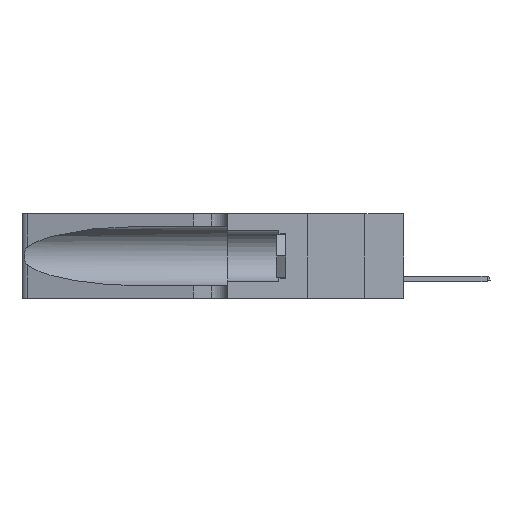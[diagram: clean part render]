
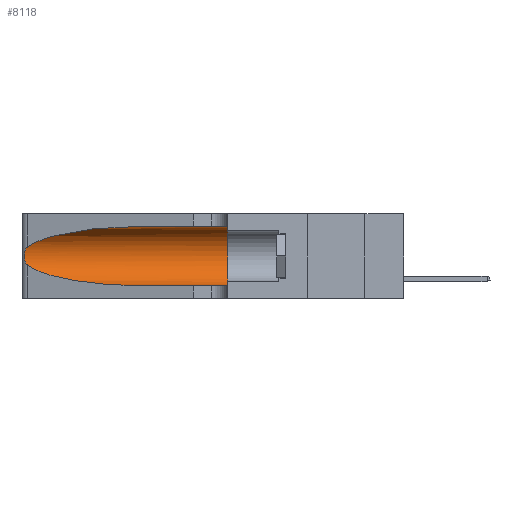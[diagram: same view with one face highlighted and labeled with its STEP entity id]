
A CAD part, left-side view. The second image highlights one B-rep face of the part: STEP entity #8118.
In plain terms, the highlighted cylindrical face has radius 3.308 mm (diameter 6.617 mm), a partial arc.
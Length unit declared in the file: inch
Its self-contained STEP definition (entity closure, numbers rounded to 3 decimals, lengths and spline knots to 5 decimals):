
#2579 = DIRECTION ( 'NONE',  ( 0., 1., 0. ) ) ;
#3588 = CARTESIAN_POINT ( 'NONE',  ( 0.1305, 0.72297, 0.05475 ) ) ;
#4040 = CARTESIAN_POINT ( 'NONE',  ( 0.1305, 0.72297, 0.31525 ) ) ;
#5181 = VECTOR ( 'NONE', #47254, 39.37008 ) ;
#6050 = CARTESIAN_POINT ( 'NONE',  ( 0.1305, 0.72297, 0.05475 ) ) ;
#7114 = EDGE_CURVE ( 'NONE', #20195, #26849, #46131, .T. ) ;
#7661 = CARTESIAN_POINT ( 'NONE',  ( 0.25639, 1.23186, 0.15144 ) ) ;
#7807 = CARTESIAN_POINT ( 'NONE',  ( 0.25555, 1.22994, 0.2215 ) ) ;
#8118 = ADVANCED_FACE ( 'NONE', ( #21408 ), #11809, .F. ) ;
#10130 = DIRECTION ( 'NONE',  ( 0., -1., 0. ) ) ;
#10303 = DIRECTION ( 'NONE',  ( 0., 0., -1. ) ) ;
#10623 = LINE ( 'NONE', #37215, #5181 ) ;
#10801 = CARTESIAN_POINT ( 'NONE',  ( 0.1305, 1.61858, 0.185 ) ) ;
#11359 = AXIS2_PLACEMENT_3D ( 'NONE', #10801, #10130, #10303 ) ;
#11375 = CARTESIAN_POINT ( 'NONE',  ( 0.26018, 1.23835, 0.19895 ) ) ;
#11809 = CYLINDRICAL_SURFACE ( 'NONE', #11359, 0.13025 ) ;
#12866 = EDGE_CURVE ( 'NONE', #38710, #25687, #27312, .T. ) ;
#13555 = EDGE_CURVE ( 'NONE', #47282, #38710, #10623, .T. ) ;
#14441 = CARTESIAN_POINT ( 'NONE',  ( 0.1305, 0.35, 0.185 ) ) ;
#15513 = CARTESIAN_POINT ( 'NONE',  ( 0.25555, 1.22993, 0.14849 ) ) ;
#16202 = ORIENTED_EDGE ( 'NONE', *, *, #36908, .T. ) ;
#17821 = VERTEX_POINT ( 'NONE', #40874 ) ;
#18726 = CARTESIAN_POINT ( 'NONE',  ( 0.26075, 1.23896, 0.178 ) ) ;
#18804 = CARTESIAN_POINT ( 'NONE',  ( 0.25487, 1.22718, 0.14631 ) ) ;
#19096 = CARTESIAN_POINT ( 'NONE',  ( 0.25487, 1.22718, 0.14631 ) ) ;
#19458 = CARTESIAN_POINT ( 'NONE',  ( 0.1305, 0.72297, 0.31525 ) ) ;
#20195 = VERTEX_POINT ( 'NONE', #19096 ) ;
#20687 = EDGE_CURVE ( 'NONE', #26849, #25687, #41101, .T. ) ;
#20751 = ORIENTED_EDGE ( 'NONE', *, *, #41582, .T. ) ;
#21408 = FACE_OUTER_BOUND ( 'NONE', #22323, .T. ) ;
#21809 = ORIENTED_EDGE ( 'NONE', *, *, #7114, .T. ) ;
#21927 = DIRECTION ( 'NONE',  ( 0., -1., 0. ) ) ;
#22323 = EDGE_LOOP ( 'NONE', ( #16202, #20751, #21809, #41801, #33899, #41941 ) ) ;
#22725 = CARTESIAN_POINT ( 'NONE',  ( 0.26017, 1.23833, 0.17102 ) ) ;
#24519 = CARTESIAN_POINT ( 'NONE',  ( 0.25487, 1.22718, 0.22369 ) ) ;
#25687 = VERTEX_POINT ( 'NONE', #37217 ) ;
#26424 = CARTESIAN_POINT ( 'NONE',  ( 0.18966, 0.96281, 0.05475 ) ) ;
#26512 = CARTESIAN_POINT ( 'NONE',  ( 0.25854, 1.2359, 0.20912 ) ) ;
#26849 = VERTEX_POINT ( 'NONE', #6050 ) ;
#26874 = CARTESIAN_POINT ( 'NONE',  ( 0.2373, 1.15595, 0.28018 ) ) ;
#27312 = CIRCLE ( 'NONE', #49216, 0.13025 ) ;
#30634 = CARTESIAN_POINT ( 'NONE',  ( 0.25487, 1.22718, 0.22369 ) ) ;
#32084 =( BOUNDED_CURVE ( )  B_SPLINE_CURVE ( 3, ( #19458, #46316, #26874, #24519 ),
 .UNSPECIFIED., .F., .T. ) 
 B_SPLINE_CURVE_WITH_KNOTS ( ( 4, 4 ),
 ( 1.5708, 2.84003 ),
 .UNSPECIFIED. ) 
 CURVE ( )  GEOMETRIC_REPRESENTATION_ITEM ( )  RATIONAL_B_SPLINE_CURVE ( ( 1., 0.87, 0.87, 1. ) ) 
 REPRESENTATION_ITEM ( '' )  );
#32607 = CARTESIAN_POINT ( 'NONE',  ( 0.1305, 0.35, 0.31525 ) ) ;
#33233 = CARTESIAN_POINT ( 'NONE',  ( 0.1305, 1.61858, 0.05475 ) ) ;
#33868 = CARTESIAN_POINT ( 'NONE',  ( 0.25639, 1.23184, 0.21858 ) ) ;
#33899 = ORIENTED_EDGE ( 'NONE', *, *, #12866, .F. ) ;
#36908 = EDGE_CURVE ( 'NONE', #47282, #17821, #32084, .T. ) ;
#37215 = CARTESIAN_POINT ( 'NONE',  ( 0.1305, 1.61858, 0.31525 ) ) ;
#37217 = CARTESIAN_POINT ( 'NONE',  ( 0.1305, 0.35, 0.05475 ) ) ;
#38016 = CARTESIAN_POINT ( 'NONE',  ( 0.25856, 1.23593, 0.16098 ) ) ;
#38341 = CARTESIAN_POINT ( 'NONE',  ( 0.25787, 1.23484, 0.2124 ) ) ;
#38710 = VERTEX_POINT ( 'NONE', #32607 ) ;
#40874 = CARTESIAN_POINT ( 'NONE',  ( 0.25487, 1.22718, 0.22369 ) ) ;
#41099 = DIRECTION ( 'NONE',  ( 0., 0., 1. ) ) ;
#41101 = LINE ( 'NONE', #33233, #45255 ) ;
#41582 = EDGE_CURVE ( 'NONE', #17821, #20195, #41600, .T. ) ;
#41600 = B_SPLINE_CURVE_WITH_KNOTS ( 'NONE', 3,
 ( #30634, #7807, #33868, #38341, #26512, #11375, #41728, #18726, #22725, #38016, #41877, #7661, #15513, #42026 ),
 .UNSPECIFIED., .F., .F.,
 ( 4, 2, 2, 2, 2, 2, 4 ),
 ( 0., 0.00027, 0.00053, 0.00107, 0.0016, 0.00187, 0.00214 ),
 .UNSPECIFIED. ) ;
#41728 = CARTESIAN_POINT ( 'NONE',  ( 0.26075, 1.23896, 0.19203 ) ) ;
#41801 = ORIENTED_EDGE ( 'NONE', *, *, #20687, .T. ) ;
#41877 = CARTESIAN_POINT ( 'NONE',  ( 0.25789, 1.23486, 0.15765 ) ) ;
#41941 = ORIENTED_EDGE ( 'NONE', *, *, #13555, .F. ) ;
#42026 = CARTESIAN_POINT ( 'NONE',  ( 0.25487, 1.22718, 0.14631 ) ) ;
#45255 = VECTOR ( 'NONE', #21927, 39.37008 ) ;
#45480 = CARTESIAN_POINT ( 'NONE',  ( 0.2373, 1.15595, 0.08982 ) ) ;
#46131 =( BOUNDED_CURVE ( )  B_SPLINE_CURVE ( 3, ( #18804, #45480, #26424, #3588 ),
 .UNSPECIFIED., .F., .T. ) 
 B_SPLINE_CURVE_WITH_KNOTS ( ( 4, 4 ),
 ( 3.44316, 4.71239 ),
 .UNSPECIFIED. ) 
 CURVE ( )  GEOMETRIC_REPRESENTATION_ITEM ( )  RATIONAL_B_SPLINE_CURVE ( ( 1., 0.87, 0.87, 1. ) ) 
 REPRESENTATION_ITEM ( '' )  );
#46316 = CARTESIAN_POINT ( 'NONE',  ( 0.18966, 0.96281, 0.31525 ) ) ;
#47254 = DIRECTION ( 'NONE',  ( 0., -1., 0. ) ) ;
#47282 = VERTEX_POINT ( 'NONE', #4040 ) ;
#49216 = AXIS2_PLACEMENT_3D ( 'NONE', #14441, #2579, #41099 ) ;
